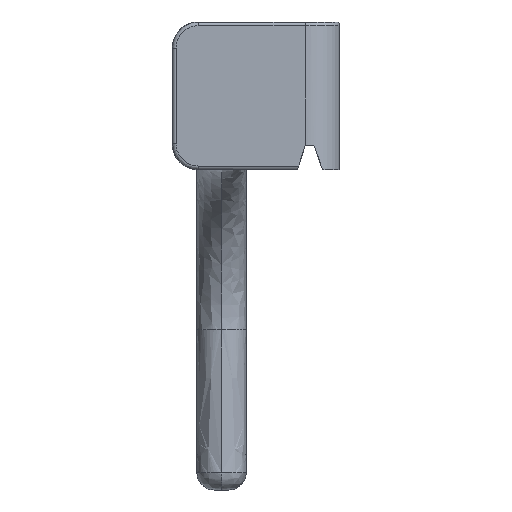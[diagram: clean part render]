
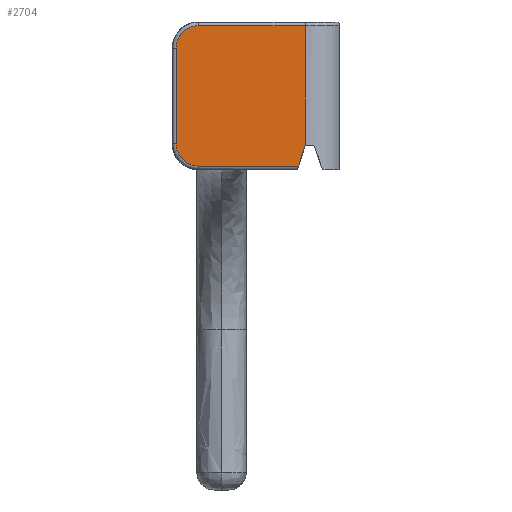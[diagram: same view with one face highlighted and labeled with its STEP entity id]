
A CAD part, front view. The second image highlights one B-rep face of the part: STEP entity #2704.
In plain terms, the highlighted planar face has unit normal (0, -1, 0).
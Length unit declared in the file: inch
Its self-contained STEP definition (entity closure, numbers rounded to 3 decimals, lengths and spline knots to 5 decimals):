
#149=PLANE('',#2881);
#297=LINE('',#6997,#453);
#298=LINE('',#7001,#454);
#299=LINE('',#7010,#455);
#300=LINE('',#7018,#456);
#301=LINE('',#7019,#457);
#453=VECTOR('',#3344,0.3937);
#454=VECTOR('',#3347,0.3937);
#455=VECTOR('',#3348,0.3937);
#456=VECTOR('',#3349,0.3937);
#457=VECTOR('',#3350,0.3937);
#636=FACE_OUTER_BOUND('',#798,.T.);
#798=EDGE_LOOP('',(#2463,#2464,#2465,#2466,#2467,#2468,#2469));
#991=B_SPLINE_CURVE_WITH_KNOTS('',3,(#7003,#7004,#7005,#7006,#7007,#7008),
 .UNSPECIFIED.,.F.,.F.,(4,1,1,4),(-0.71331,-0.40761,
-0.2038,0.),.UNSPECIFIED.);
#992=B_SPLINE_CURVE_WITH_KNOTS('',3,(#7012,#7013,#7014,#7015,#7016,#7017),
 .UNSPECIFIED.,.F.,.F.,(4,1,1,4),(-0.71331,-0.50951,
-0.3057,0.),.UNSPECIFIED.);
#1290=VERTEX_POINT('',#6962);
#1300=VERTEX_POINT('',#6994);
#1301=VERTEX_POINT('',#6999);
#1302=VERTEX_POINT('',#7000);
#1303=VERTEX_POINT('',#7002);
#1304=VERTEX_POINT('',#7009);
#1305=VERTEX_POINT('',#7011);
#1699=EDGE_CURVE('',#1300,#1290,#297,.T.);
#1700=EDGE_CURVE('',#1301,#1302,#298,.T.);
#1701=EDGE_CURVE('',#1303,#1301,#991,.T.);
#1702=EDGE_CURVE('',#1304,#1303,#299,.T.);
#1703=EDGE_CURVE('',#1305,#1304,#992,.T.);
#1704=EDGE_CURVE('',#1300,#1305,#300,.T.);
#1705=EDGE_CURVE('',#1302,#1290,#301,.T.);
#2463=ORIENTED_EDGE('',*,*,#1700,.F.);
#2464=ORIENTED_EDGE('',*,*,#1701,.F.);
#2465=ORIENTED_EDGE('',*,*,#1702,.F.);
#2466=ORIENTED_EDGE('',*,*,#1703,.F.);
#2467=ORIENTED_EDGE('',*,*,#1704,.F.);
#2468=ORIENTED_EDGE('',*,*,#1699,.T.);
#2469=ORIENTED_EDGE('',*,*,#1705,.F.);
#2704=ADVANCED_FACE('',(#636),#149,.T.);
#2881=AXIS2_PLACEMENT_3D('',#6998,#3345,#3346);
#3344=DIRECTION('',(0.3,0.,0.954));
#3345=DIRECTION('center_axis',(0.,-1.,0.));
#3346=DIRECTION('ref_axis',(0.,0.,
-1.));
#3347=DIRECTION('',(1.,0.,0.));
#3348=DIRECTION('',(0.,0.,1.));
#3349=DIRECTION('',(-1.,0.,0.));
#3350=DIRECTION('',(0.,0.,-1.));
#6962=CARTESIAN_POINT('',(0.6717,3.13929,-2.02348));
#6994=CARTESIAN_POINT('',(0.61918,3.13929,-2.19033));
#6997=CARTESIAN_POINT('',(0.74261,3.13929,-1.79815));
#6998=CARTESIAN_POINT('Origin',(-0.19445,3.13929,-1.03923));
#6999=CARTESIAN_POINT('',(-0.18251,3.13929,-1.06923));
#7000=CARTESIAN_POINT('',(0.6717,3.13929,-1.06923));
#7001=CARTESIAN_POINT('',(-0.19445,3.13929,-1.06923));
#7002=CARTESIAN_POINT('',(-0.3613,3.13929,-1.24802));
#7003=CARTESIAN_POINT('Ctrl Pts',(-0.3613,3.13929,-1.24802));
#7004=CARTESIAN_POINT('Ctrl Pts',(-0.3613,3.13929,-1.2079));
#7005=CARTESIAN_POINT('Ctrl Pts',(-0.33784,3.13929,-1.14128));
#7006=CARTESIAN_POINT('Ctrl Pts',(-0.26264,3.13929,-1.08147));
#7007=CARTESIAN_POINT('Ctrl Pts',(-0.20925,3.13929,-1.06923));
#7008=CARTESIAN_POINT('Ctrl Pts',(-0.18251,3.13929,-1.06923));
#7009=CARTESIAN_POINT('',(-0.3613,3.13929,-2.01154));
#7010=CARTESIAN_POINT('',(-0.3613,3.13929,-1.97427));
#7011=CARTESIAN_POINT('',(-0.18251,3.13929,-2.19033));
#7012=CARTESIAN_POINT('Ctrl Pts',(-0.18251,3.13929,-2.19033));
#7013=CARTESIAN_POINT('Ctrl Pts',(-0.20925,3.13929,-2.19033));
#7014=CARTESIAN_POINT('Ctrl Pts',(-0.26264,3.13929,-2.17809));
#7015=CARTESIAN_POINT('Ctrl Pts',(-0.33783,3.13929,-2.11828));
#7016=CARTESIAN_POINT('Ctrl Pts',(-0.3613,3.13929,-2.05166));
#7017=CARTESIAN_POINT('Ctrl Pts',(-0.3613,3.13929,-2.01154));
#7018=CARTESIAN_POINT('',(-0.19445,3.13929,-2.19033));
#7019=CARTESIAN_POINT('',(0.6717,3.13929,-1.3345));
